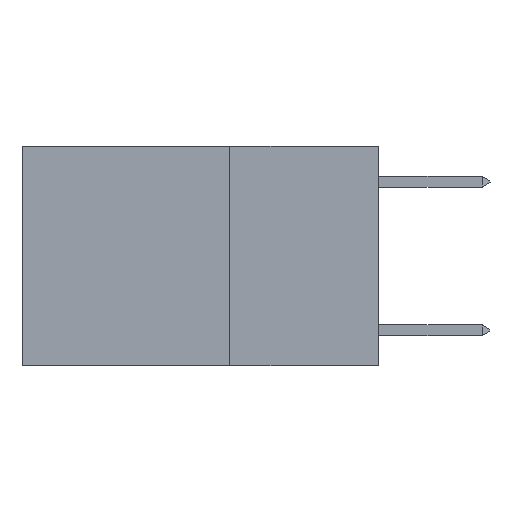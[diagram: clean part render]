
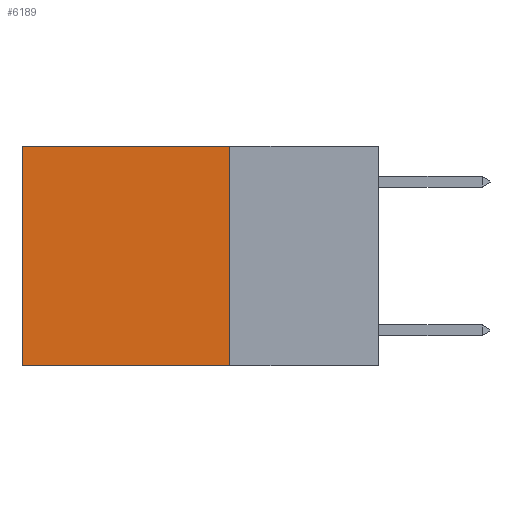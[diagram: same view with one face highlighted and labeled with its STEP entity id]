
A CAD part, left-side view. The second image highlights one B-rep face of the part: STEP entity #6189.
In plain terms, the highlighted planar face has unit normal (-1, 0, 0).
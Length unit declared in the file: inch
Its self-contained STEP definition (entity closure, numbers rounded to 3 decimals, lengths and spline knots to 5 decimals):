
#968 = CARTESIAN_POINT ( 'NONE',  ( 0.2625, 0.25, 0. ) ) ;
#1073 = DIRECTION ( 'NONE',  ( 0., 0., -1. ) ) ;
#1331 = DIRECTION ( 'NONE',  ( 0., 0., -1. ) ) ;
#3475 = FACE_OUTER_BOUND ( 'NONE', #19278, .T. ) ;
#4297 = PLANE ( 'NONE',  #5749 ) ;
#4753 = ORIENTED_EDGE ( 'NONE', *, *, #7020, .F. ) ;
#5749 = AXIS2_PLACEMENT_3D ( 'NONE', #19870, #6494, #22141 ) ;
#6189 = ADVANCED_FACE ( 'NONE', ( #3475 ), #4297, .F. ) ;
#6494 = DIRECTION ( 'NONE',  ( 1., 0., 0. ) ) ;
#7020 = EDGE_CURVE ( 'NONE', #24603, #24725, #15152, .T. ) ;
#7280 = VECTOR ( 'NONE', #1331, 39.37008 ) ;
#7548 = LINE ( 'NONE', #19080, #7280 ) ;
#7855 = VERTEX_POINT ( 'NONE', #23446 ) ;
#8248 = ORIENTED_EDGE ( 'NONE', *, *, #21281, .T. ) ;
#9410 = CARTESIAN_POINT ( 'NONE',  ( 0.2625, 0.25, -0.37 ) ) ;
#11269 = VERTEX_POINT ( 'NONE', #968 ) ;
#11424 = EDGE_CURVE ( 'NONE', #7855, #24725, #7548, .T. ) ;
#11795 = ORIENTED_EDGE ( 'NONE', *, *, #22626, .F. ) ;
#12032 = CARTESIAN_POINT ( 'NONE',  ( 0.2625, 0.6, -0.37 ) ) ;
#12143 = CARTESIAN_POINT ( 'NONE',  ( 0.2625, 0.25, 0. ) ) ;
#12401 = VECTOR ( 'NONE', #23293, 39.37008 ) ;
#13028 = VECTOR ( 'NONE', #1073, 39.37008 ) ;
#14855 = VECTOR ( 'NONE', #22671, 39.37008 ) ;
#15152 = LINE ( 'NONE', #15875, #14855 ) ;
#15875 = CARTESIAN_POINT ( 'NONE',  ( 0.2625, 0.25, -0.37 ) ) ;
#16456 = CARTESIAN_POINT ( 'NONE',  ( 0.2625, 0.25, 0. ) ) ;
#19048 = LINE ( 'NONE', #12143, #12401 ) ;
#19080 = CARTESIAN_POINT ( 'NONE',  ( 0.2625, 0.6, 0. ) ) ;
#19278 = EDGE_LOOP ( 'NONE', ( #26514, #4753, #11795, #8248 ) ) ;
#19735 = LINE ( 'NONE', #16456, #13028 ) ;
#19870 = CARTESIAN_POINT ( 'NONE',  ( 0.2625, 0.25, 0. ) ) ;
#21281 = EDGE_CURVE ( 'NONE', #11269, #7855, #19048, .T. ) ;
#22141 = DIRECTION ( 'NONE',  ( 0., 0., -1. ) ) ;
#22626 = EDGE_CURVE ( 'NONE', #11269, #24603, #19735, .T. ) ;
#22671 = DIRECTION ( 'NONE',  ( 0., 1., 0. ) ) ;
#23293 = DIRECTION ( 'NONE',  ( 0., 1., 0. ) ) ;
#23446 = CARTESIAN_POINT ( 'NONE',  ( 0.2625, 0.6, 0. ) ) ;
#24603 = VERTEX_POINT ( 'NONE', #9410 ) ;
#24725 = VERTEX_POINT ( 'NONE', #12032 ) ;
#26514 = ORIENTED_EDGE ( 'NONE', *, *, #11424, .T. ) ;
